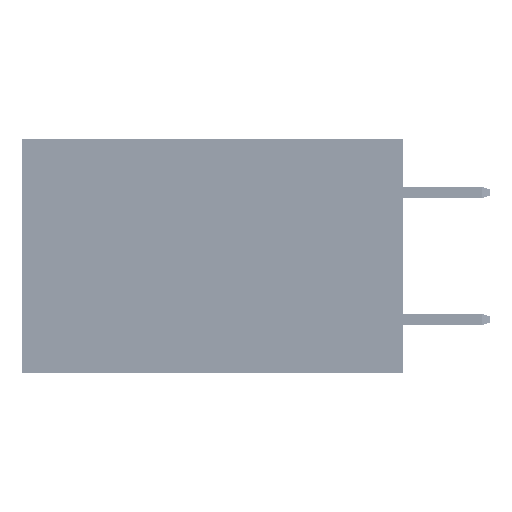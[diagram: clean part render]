
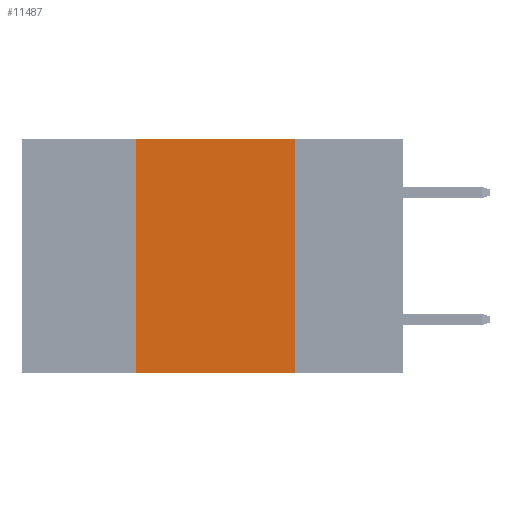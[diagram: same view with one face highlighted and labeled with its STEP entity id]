
A CAD part, left-side view. The second image highlights one B-rep face of the part: STEP entity #11487.
In plain terms, the highlighted planar face has unit normal (-1, 0, 0).
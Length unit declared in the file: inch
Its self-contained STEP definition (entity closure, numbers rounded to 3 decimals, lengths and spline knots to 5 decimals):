
#3201 = EDGE_LOOP ( 'NONE', ( #31205, #19772, #6161, #29755 ) ) ;
#4686 = LINE ( 'NONE', #5185, #44324 ) ;
#5185 = CARTESIAN_POINT ( 'NONE',  ( 0., 0.6, -0.37 ) ) ;
#6161 = ORIENTED_EDGE ( 'NONE', *, *, #43962, .F. ) ;
#7510 = VECTOR ( 'NONE', #12762, 39.37008 ) ;
#9559 = CARTESIAN_POINT ( 'NONE',  ( 0., 0.17, 0. ) ) ;
#10143 = EDGE_CURVE ( 'NONE', #37081, #22972, #4686, .T. ) ;
#11487 = ADVANCED_FACE ( 'NONE', ( #28854 ), #40446, .F. ) ;
#12762 = DIRECTION ( 'NONE',  ( 0., -1., 0. ) ) ;
#14949 = CARTESIAN_POINT ( 'NONE',  ( 0., 0.17, -0.37 ) ) ;
#19714 = CARTESIAN_POINT ( 'NONE',  ( 0., 0.6, 0. ) ) ;
#19772 = ORIENTED_EDGE ( 'NONE', *, *, #50492, .F. ) ;
#20741 = VECTOR ( 'NONE', #28610, 39.37008 ) ;
#20886 = VERTEX_POINT ( 'NONE', #25809 ) ;
#22972 = VERTEX_POINT ( 'NONE', #14949 ) ;
#23791 = AXIS2_PLACEMENT_3D ( 'NONE', #44528, #32474, #43763 ) ;
#25809 = CARTESIAN_POINT ( 'NONE',  ( 0., 0.42, 0. ) ) ;
#28486 = LINE ( 'NONE', #33116, #34199 ) ;
#28610 = DIRECTION ( 'NONE',  ( 0., 0., -1. ) ) ;
#28854 = FACE_OUTER_BOUND ( 'NONE', #3201, .T. ) ;
#29755 = ORIENTED_EDGE ( 'NONE', *, *, #10143, .T. ) ;
#31205 = ORIENTED_EDGE ( 'NONE', *, *, #39338, .F. ) ;
#32474 = DIRECTION ( 'NONE',  ( 1., 0., 0. ) ) ;
#33116 = CARTESIAN_POINT ( 'NONE',  ( 0., 0.42, 0. ) ) ;
#34199 = VECTOR ( 'NONE', #48772, 39.37008 ) ;
#35567 = LINE ( 'NONE', #43525, #20741 ) ;
#37081 = VERTEX_POINT ( 'NONE', #46575 ) ;
#39338 = EDGE_CURVE ( 'NONE', #49880, #22972, #35567, .T. ) ;
#40298 = LINE ( 'NONE', #19714, #7510 ) ;
#40446 = PLANE ( 'NONE',  #23791 ) ;
#43525 = CARTESIAN_POINT ( 'NONE',  ( 0., 0.17, 0. ) ) ;
#43763 = DIRECTION ( 'NONE',  ( 0., 0., -1. ) ) ;
#43962 = EDGE_CURVE ( 'NONE', #37081, #20886, #28486, .T. ) ;
#44015 = DIRECTION ( 'NONE',  ( 0., -1., 0. ) ) ;
#44324 = VECTOR ( 'NONE', #44015, 39.37008 ) ;
#44528 = CARTESIAN_POINT ( 'NONE',  ( 0., 0.6, 0. ) ) ;
#46575 = CARTESIAN_POINT ( 'NONE',  ( 0., 0.42, -0.37 ) ) ;
#48772 = DIRECTION ( 'NONE',  ( 0., 0., 1. ) ) ;
#49880 = VERTEX_POINT ( 'NONE', #9559 ) ;
#50492 = EDGE_CURVE ( 'NONE', #20886, #49880, #40298, .T. ) ;
